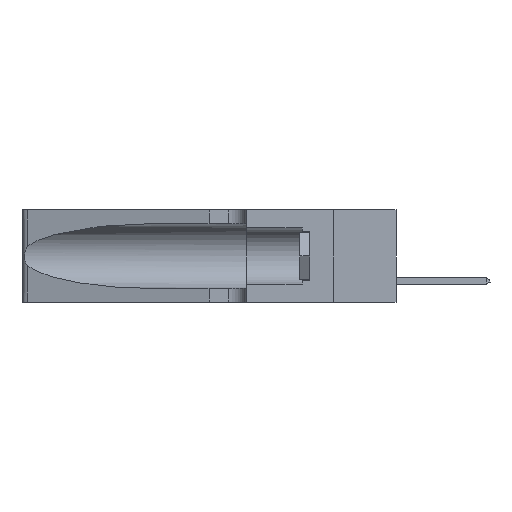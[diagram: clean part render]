
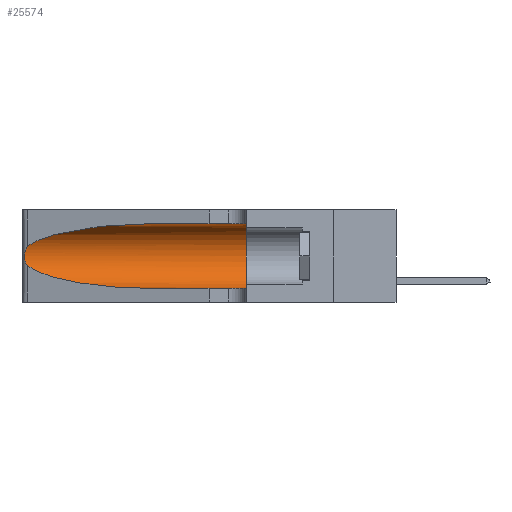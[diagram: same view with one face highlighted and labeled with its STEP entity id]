
A CAD part, left-side view. The second image highlights one B-rep face of the part: STEP entity #25574.
In plain terms, the highlighted cylindrical face has radius 3.308 mm (diameter 6.617 mm), a partial arc.
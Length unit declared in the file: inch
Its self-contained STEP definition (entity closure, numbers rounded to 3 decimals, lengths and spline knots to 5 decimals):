
#301 = ORIENTED_EDGE ( 'NONE', *, *, #4783, .T. ) ;
#586 = LINE ( 'NONE', #21681, #19325 ) ;
#1161 = FACE_OUTER_BOUND ( 'NONE', #13387, .T. ) ;
#1944 = VERTEX_POINT ( 'NONE', #25230 ) ;
#2121 = AXIS2_PLACEMENT_3D ( 'NONE', #41169, #16989, #48963 ) ;
#2447 = CARTESIAN_POINT ( 'NONE',  ( 0.25487, 1.22718, 0.22369 ) ) ;
#2459 = DIRECTION ( 'NONE',  ( 0., 0., -1. ) ) ;
#3132 = VERTEX_POINT ( 'NONE', #18824 ) ;
#3659 = ORIENTED_EDGE ( 'NONE', *, *, #10283, .F. ) ;
#4033 = DIRECTION ( 'NONE',  ( 0., -1., 0. ) ) ;
#4783 = EDGE_CURVE ( 'NONE', #5958, #25808, #41926, .T. ) ;
#5620 = ORIENTED_EDGE ( 'NONE', *, *, #33078, .T. ) ;
#5958 = VERTEX_POINT ( 'NONE', #49814 ) ;
#6256 = VERTEX_POINT ( 'NONE', #14845 ) ;
#6427 = CARTESIAN_POINT ( 'NONE',  ( 0.26075, 1.23896, 0.19203 ) ) ;
#6599 = CARTESIAN_POINT ( 'NONE',  ( 0.25789, 1.23486, 0.15765 ) ) ;
#10283 = EDGE_CURVE ( 'NONE', #1944, #3132, #30552, .T. ) ;
#10400 = CARTESIAN_POINT ( 'NONE',  ( 0.26075, 1.23896, 0.178 ) ) ;
#12364 =( BOUNDED_CURVE ( )  B_SPLINE_CURVE ( 3, ( #45041, #25123, #21276, #18129 ),
 .UNSPECIFIED., .F., .F. ) 
 B_SPLINE_CURVE_WITH_KNOTS ( ( 4, 4 ),
 ( 1.5708, 2.84003 ),
 .UNSPECIFIED. ) 
 CURVE ( )  GEOMETRIC_REPRESENTATION_ITEM ( )  RATIONAL_B_SPLINE_CURVE ( ( 1., 0.87, 0.87, 1. ) ) 
 REPRESENTATION_ITEM ( '' )  );
#13387 = EDGE_LOOP ( 'NONE', ( #17964, #301, #5620, #28875, #3659, #44676 ) ) ;
#14416 = CARTESIAN_POINT ( 'NONE',  ( 0.26017, 1.23833, 0.17102 ) ) ;
#14786 = DIRECTION ( 'NONE',  ( 0., -1., 0. ) ) ;
#14845 = CARTESIAN_POINT ( 'NONE',  ( 0.1305, 0.72297, 0.31525 ) ) ;
#16989 = DIRECTION ( 'NONE',  ( 0., 1., 0. ) ) ;
#17101 = DIRECTION ( 'NONE',  ( 0., -1., 0. ) ) ;
#17231 = VERTEX_POINT ( 'NONE', #30605 ) ;
#17964 = ORIENTED_EDGE ( 'NONE', *, *, #35182, .T. ) ;
#18129 = CARTESIAN_POINT ( 'NONE',  ( 0.25487, 1.22718, 0.22369 ) ) ;
#18430 = CARTESIAN_POINT ( 'NONE',  ( 0.25856, 1.23593, 0.16098 ) ) ;
#18824 = CARTESIAN_POINT ( 'NONE',  ( 0.1305, 0.35, 0.05475 ) ) ;
#19325 = VECTOR ( 'NONE', #17101, 39.37008 ) ;
#20147 = LINE ( 'NONE', #30973, #42111 ) ;
#21276 = CARTESIAN_POINT ( 'NONE',  ( 0.2373, 1.15595, 0.28018 ) ) ;
#21681 = CARTESIAN_POINT ( 'NONE',  ( 0.1305, 1.61858, 0.05475 ) ) ;
#22297 = CARTESIAN_POINT ( 'NONE',  ( 0.25787, 1.23484, 0.2124 ) ) ;
#22761 = CARTESIAN_POINT ( 'NONE',  ( 0.1305, 0.72297, 0.05475 ) ) ;
#23503 = EDGE_CURVE ( 'NONE', #6256, #1944, #20147, .T. ) ;
#25123 = CARTESIAN_POINT ( 'NONE',  ( 0.18966, 0.96281, 0.31525 ) ) ;
#25230 = CARTESIAN_POINT ( 'NONE',  ( 0.1305, 0.35, 0.31525 ) ) ;
#25574 = ADVANCED_FACE ( 'NONE', ( #1161 ), #42481, .F. ) ;
#25808 = VERTEX_POINT ( 'NONE', #42772 ) ;
#26319 = CARTESIAN_POINT ( 'NONE',  ( 0.26018, 1.23835, 0.19895 ) ) ;
#28396 = CARTESIAN_POINT ( 'NONE',  ( 0.25555, 1.22993, 0.14849 ) ) ;
#28875 = ORIENTED_EDGE ( 'NONE', *, *, #42837, .T. ) ;
#30104 = CARTESIAN_POINT ( 'NONE',  ( 0.25487, 1.22718, 0.14631 ) ) ;
#30552 = CIRCLE ( 'NONE', #2121, 0.13025 ) ;
#30605 = CARTESIAN_POINT ( 'NONE',  ( 0.1305, 0.72297, 0.05475 ) ) ;
#30681 = AXIS2_PLACEMENT_3D ( 'NONE', #33724, #14786, #2459 ) ;
#30973 = CARTESIAN_POINT ( 'NONE',  ( 0.1305, 1.61858, 0.31525 ) ) ;
#33078 = EDGE_CURVE ( 'NONE', #25808, #17231, #37098, .T. ) ;
#33724 = CARTESIAN_POINT ( 'NONE',  ( 0.1305, 1.61858, 0.185 ) ) ;
#33994 = CARTESIAN_POINT ( 'NONE',  ( 0.25487, 1.22718, 0.14631 ) ) ;
#34668 = CARTESIAN_POINT ( 'NONE',  ( 0.18966, 0.96281, 0.05475 ) ) ;
#35182 = EDGE_CURVE ( 'NONE', #6256, #5958, #12364, .T. ) ;
#37098 =( BOUNDED_CURVE ( )  B_SPLINE_CURVE ( 3, ( #30104, #50305, #34668, #22761 ),
 .UNSPECIFIED., .F., .F. ) 
 B_SPLINE_CURVE_WITH_KNOTS ( ( 4, 4 ),
 ( 3.44316, 4.71239 ),
 .UNSPECIFIED. ) 
 CURVE ( )  GEOMETRIC_REPRESENTATION_ITEM ( )  RATIONAL_B_SPLINE_CURVE ( ( 1., 0.87, 0.87, 1. ) ) 
 REPRESENTATION_ITEM ( '' )  );
#41169 = CARTESIAN_POINT ( 'NONE',  ( 0.1305, 0.35, 0.185 ) ) ;
#41718 = CARTESIAN_POINT ( 'NONE',  ( 0.25555, 1.22994, 0.2215 ) ) ;
#41926 = B_SPLINE_CURVE_WITH_KNOTS ( 'NONE', 3,
 ( #2447, #41718, #46221, #22297, #50225, #26319, #6427, #10400, #14416, #18430, #6599, #47763, #28396, #33994 ),
 .UNSPECIFIED., .F., .F.,
 ( 4, 2, 2, 2, 2, 2, 4 ),
 ( 0., 0.00027, 0.00053, 0.00107, 0.0016, 0.00187, 0.00214 ),
 .UNSPECIFIED. ) ;
#42111 = VECTOR ( 'NONE', #4033, 39.37008 ) ;
#42481 = CYLINDRICAL_SURFACE ( 'NONE', #30681, 0.13025 ) ;
#42772 = CARTESIAN_POINT ( 'NONE',  ( 0.25487, 1.22718, 0.14631 ) ) ;
#42837 = EDGE_CURVE ( 'NONE', #17231, #3132, #586, .T. ) ;
#44676 = ORIENTED_EDGE ( 'NONE', *, *, #23503, .F. ) ;
#45041 = CARTESIAN_POINT ( 'NONE',  ( 0.1305, 0.72297, 0.31525 ) ) ;
#46221 = CARTESIAN_POINT ( 'NONE',  ( 0.25639, 1.23184, 0.21858 ) ) ;
#47763 = CARTESIAN_POINT ( 'NONE',  ( 0.25639, 1.23186, 0.15144 ) ) ;
#48963 = DIRECTION ( 'NONE',  ( 0., 0., 1. ) ) ;
#49814 = CARTESIAN_POINT ( 'NONE',  ( 0.25487, 1.22718, 0.22369 ) ) ;
#50225 = CARTESIAN_POINT ( 'NONE',  ( 0.25854, 1.2359, 0.20912 ) ) ;
#50305 = CARTESIAN_POINT ( 'NONE',  ( 0.2373, 1.15595, 0.08982 ) ) ;
